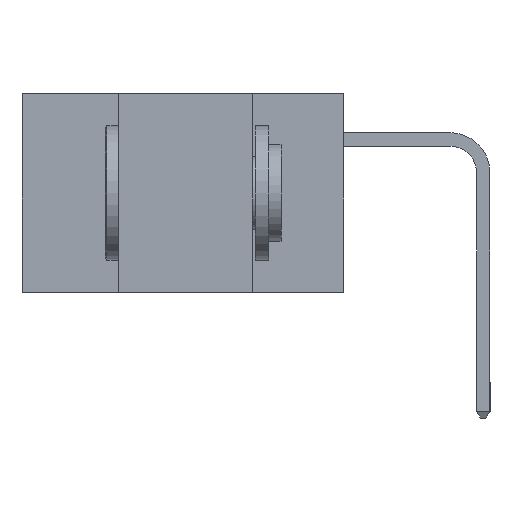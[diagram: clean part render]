
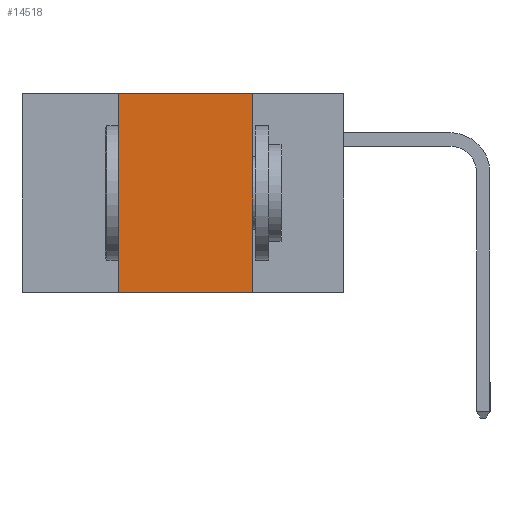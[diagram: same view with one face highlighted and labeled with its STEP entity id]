
A CAD part, left-side view. The second image highlights one B-rep face of the part: STEP entity #14518.
In plain terms, the highlighted planar face has unit normal (-1, 0, 0).
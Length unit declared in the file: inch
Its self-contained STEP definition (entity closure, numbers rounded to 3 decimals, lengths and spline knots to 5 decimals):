
#522 = DIRECTION ( 'NONE',  ( 0., -1., 0. ) ) ;
#853 = ORIENTED_EDGE ( 'NONE', *, *, #4978, .F. ) ;
#1241 = EDGE_CURVE ( 'NONE', #15830, #21367, #1918, .T. ) ;
#1724 = VERTEX_POINT ( 'NONE', #3656 ) ;
#1918 = LINE ( 'NONE', #2934, #19273 ) ;
#2484 = ORIENTED_EDGE ( 'NONE', *, *, #2661, .T. ) ;
#2632 = EDGE_LOOP ( 'NONE', ( #17783, #18299, #853, #2484 ) ) ;
#2661 = EDGE_CURVE ( 'NONE', #1724, #3277, #13344, .T. ) ;
#2934 = CARTESIAN_POINT ( 'NONE',  ( 0., 0.6, 0. ) ) ;
#3091 = LINE ( 'NONE', #6335, #11690 ) ;
#3242 = CARTESIAN_POINT ( 'NONE',  ( 0., 0.6, -0.37 ) ) ;
#3277 = VERTEX_POINT ( 'NONE', #17970 ) ;
#3656 = CARTESIAN_POINT ( 'NONE',  ( 0., 0.42, -0.37 ) ) ;
#3886 = DIRECTION ( 'NONE',  ( 0., 0., -1. ) ) ;
#4271 = VECTOR ( 'NONE', #522, 39.37008 ) ;
#4978 = EDGE_CURVE ( 'NONE', #1724, #15830, #8374, .T. ) ;
#6194 = CARTESIAN_POINT ( 'NONE',  ( 0., 0.42, 0. ) ) ;
#6335 = CARTESIAN_POINT ( 'NONE',  ( 0., 0.17, 0. ) ) ;
#6475 = DIRECTION ( 'NONE',  ( 0., 0., -1. ) ) ;
#7274 = CARTESIAN_POINT ( 'NONE',  ( 0., 0.6, 0. ) ) ;
#8374 = LINE ( 'NONE', #6194, #12348 ) ;
#8547 = DIRECTION ( 'NONE',  ( 0., -1., 0. ) ) ;
#8731 = EDGE_CURVE ( 'NONE', #21367, #3277, #3091, .T. ) ;
#9005 = CARTESIAN_POINT ( 'NONE',  ( 0., 0.42, 0. ) ) ;
#10686 = PLANE ( 'NONE',  #14130 ) ;
#11690 = VECTOR ( 'NONE', #6475, 39.37008 ) ;
#12348 = VECTOR ( 'NONE', #21373, 39.37008 ) ;
#13344 = LINE ( 'NONE', #3242, #4271 ) ;
#14066 = DIRECTION ( 'NONE',  ( 1., 0., 0. ) ) ;
#14130 = AXIS2_PLACEMENT_3D ( 'NONE', #7274, #14066, #3886 ) ;
#14518 = ADVANCED_FACE ( 'NONE', ( #16556 ), #10686, .F. ) ;
#15435 = CARTESIAN_POINT ( 'NONE',  ( 0., 0.17, 0. ) ) ;
#15830 = VERTEX_POINT ( 'NONE', #9005 ) ;
#16556 = FACE_OUTER_BOUND ( 'NONE', #2632, .T. ) ;
#17783 = ORIENTED_EDGE ( 'NONE', *, *, #8731, .F. ) ;
#17970 = CARTESIAN_POINT ( 'NONE',  ( 0., 0.17, -0.37 ) ) ;
#18299 = ORIENTED_EDGE ( 'NONE', *, *, #1241, .F. ) ;
#19273 = VECTOR ( 'NONE', #8547, 39.37008 ) ;
#21367 = VERTEX_POINT ( 'NONE', #15435 ) ;
#21373 = DIRECTION ( 'NONE',  ( 0., 0., 1. ) ) ;
